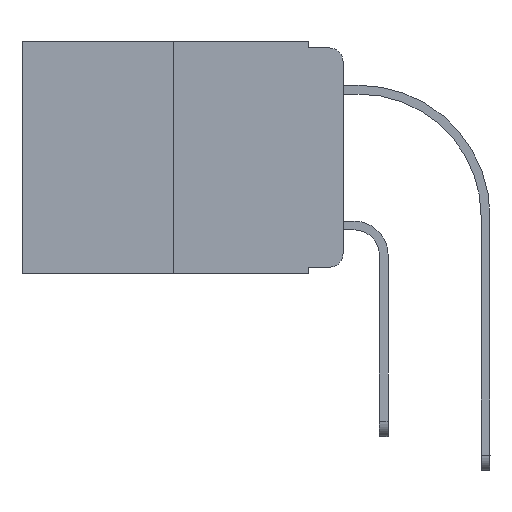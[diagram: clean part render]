
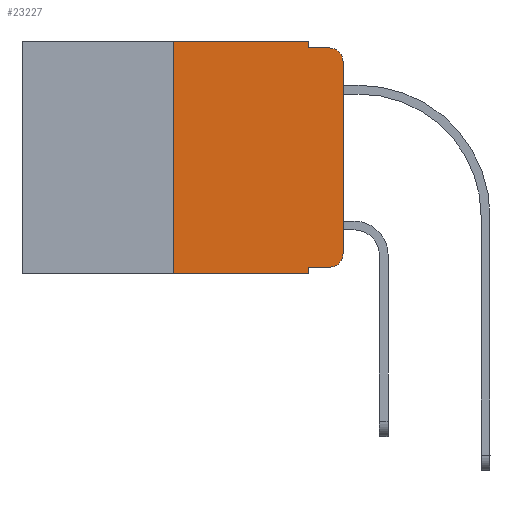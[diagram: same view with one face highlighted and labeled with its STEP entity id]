
A CAD part, left-side view. The second image highlights one B-rep face of the part: STEP entity #23227.
In plain terms, the highlighted planar face has unit normal (-1, 0, 0).
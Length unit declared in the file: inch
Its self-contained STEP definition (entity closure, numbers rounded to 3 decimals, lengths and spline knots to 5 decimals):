
#122 = EDGE_CURVE ( 'NONE', #24338, #26488, #23651, .T. ) ;
#139 = CARTESIAN_POINT ( 'NONE',  ( 0., 0.051, -0.01 ) ) ;
#524 = CARTESIAN_POINT ( 'NONE',  ( 0., 0.051, -0.01 ) ) ;
#1080 = CARTESIAN_POINT ( 'NONE',  ( 0., 0.473, 0. ) ) ;
#1432 = DIRECTION ( 'NONE',  ( 0., 0., -1. ) ) ;
#1487 = DIRECTION ( 'NONE',  ( 0., -1., 0. ) ) ;
#1565 = VECTOR ( 'NONE', #1432, 39.37008 ) ;
#1876 = DIRECTION ( 'NONE',  ( 0., 0., 1. ) ) ;
#2195 = EDGE_CURVE ( 'NONE', #5701, #9958, #22381, .T. ) ;
#2500 = VERTEX_POINT ( 'NONE', #13990 ) ;
#2612 = DIRECTION ( 'NONE',  ( 0., -1., 0. ) ) ;
#3319 = CARTESIAN_POINT ( 'NONE',  ( 0., 0.25, 0. ) ) ;
#3854 = CARTESIAN_POINT ( 'NONE',  ( 0., 0., -0.313 ) ) ;
#4149 = VERTEX_POINT ( 'NONE', #12346 ) ;
#4293 = EDGE_CURVE ( 'NONE', #4149, #24338, #19023, .T. ) ;
#4518 = CIRCLE ( 'NONE', #11486, 0.02 ) ;
#4708 = LINE ( 'NONE', #25182, #15125 ) ;
#5687 = EDGE_CURVE ( 'NONE', #6846, #24163, #4518, .T. ) ;
#5701 = VERTEX_POINT ( 'NONE', #9592 ) ;
#6397 = DIRECTION ( 'NONE',  ( 0., -1., 0. ) ) ;
#6399 = ORIENTED_EDGE ( 'NONE', *, *, #12714, .F. ) ;
#6846 = VERTEX_POINT ( 'NONE', #12774 ) ;
#7300 = DIRECTION ( 'NONE',  ( 0., 0., 1. ) ) ;
#7724 = ORIENTED_EDGE ( 'NONE', *, *, #22183, .T. ) ;
#7801 = VERTEX_POINT ( 'NONE', #10499 ) ;
#7982 = EDGE_LOOP ( 'NONE', ( #13857, #7724, #8784, #21289, #6399, #9930, #16809, #25995, #10051, #22734 ) ) ;
#8472 = VECTOR ( 'NONE', #7300, 39.37008 ) ;
#8784 = ORIENTED_EDGE ( 'NONE', *, *, #122, .F. ) ;
#9409 = DIRECTION ( 'NONE',  ( 1., 0., 0. ) ) ;
#9592 = CARTESIAN_POINT ( 'NONE',  ( 0., 0.25, -0.343 ) ) ;
#9930 = ORIENTED_EDGE ( 'NONE', *, *, #14198, .F. ) ;
#9958 = VERTEX_POINT ( 'NONE', #18833 ) ;
#10037 = DIRECTION ( 'NONE',  ( -1., 0., 0. ) ) ;
#10051 = ORIENTED_EDGE ( 'NONE', *, *, #18246, .T. ) ;
#10071 = CARTESIAN_POINT ( 'NONE',  ( 0., 0.473, -0.343 ) ) ;
#10430 = DIRECTION ( 'NONE',  ( 0., 0., -1. ) ) ;
#10499 = CARTESIAN_POINT ( 'NONE',  ( 0., 0.25, 0. ) ) ;
#10793 = CARTESIAN_POINT ( 'NONE',  ( 0., 0.051, -0.333 ) ) ;
#11015 = EDGE_CURVE ( 'NONE', #13066, #9958, #26423, .T. ) ;
#11486 = AXIS2_PLACEMENT_3D ( 'NONE', #25319, #14923, #14803 ) ;
#12346 = CARTESIAN_POINT ( 'NONE',  ( 0., 0.051, 0. ) ) ;
#12363 = CARTESIAN_POINT ( 'NONE',  ( 0., 0.02, -0.03 ) ) ;
#12500 = VECTOR ( 'NONE', #6397, 39.37008 ) ;
#12528 = LINE ( 'NONE', #18531, #12500 ) ;
#12714 = EDGE_CURVE ( 'NONE', #7801, #4149, #4708, .T. ) ;
#12774 = CARTESIAN_POINT ( 'NONE',  ( 0., 0.02, -0.333 ) ) ;
#13066 = VERTEX_POINT ( 'NONE', #10793 ) ;
#13857 = ORIENTED_EDGE ( 'NONE', *, *, #18279, .T. ) ;
#13990 = CARTESIAN_POINT ( 'NONE',  ( 0., 0., -0.03 ) ) ;
#14147 = DIRECTION ( 'NONE',  ( 0., 0., -1. ) ) ;
#14198 = EDGE_CURVE ( 'NONE', #5701, #7801, #22038, .T. ) ;
#14682 = VECTOR ( 'NONE', #1876, 39.37008 ) ;
#14803 = DIRECTION ( 'NONE',  ( 0., 0., -1. ) ) ;
#14917 = CARTESIAN_POINT ( 'NONE',  ( 0., 0.051, 0. ) ) ;
#14923 = DIRECTION ( 'NONE',  ( -1., 0., 0. ) ) ;
#15125 = VECTOR ( 'NONE', #25988, 39.37008 ) ;
#15651 = CIRCLE ( 'NONE', #21790, 0.02 ) ;
#15767 = VECTOR ( 'NONE', #1487, 39.37008 ) ;
#16355 = CARTESIAN_POINT ( 'NONE',  ( 0., 0., 0. ) ) ;
#16360 = CARTESIAN_POINT ( 'NONE',  ( 0., 0.02, -0.01 ) ) ;
#16708 = VECTOR ( 'NONE', #10430, 39.37008 ) ;
#16809 = ORIENTED_EDGE ( 'NONE', *, *, #2195, .T. ) ;
#18246 = EDGE_CURVE ( 'NONE', #13066, #6846, #12528, .T. ) ;
#18279 = EDGE_CURVE ( 'NONE', #24163, #2500, #22648, .T. ) ;
#18531 = CARTESIAN_POINT ( 'NONE',  ( 0., 0.051, -0.333 ) ) ;
#18833 = CARTESIAN_POINT ( 'NONE',  ( 0., 0.051, -0.343 ) ) ;
#19023 = LINE ( 'NONE', #14917, #16708 ) ;
#19651 = FACE_OUTER_BOUND ( 'NONE', #7982, .T. ) ;
#21289 = ORIENTED_EDGE ( 'NONE', *, *, #4293, .F. ) ;
#21790 = AXIS2_PLACEMENT_3D ( 'NONE', #12363, #10037, #14147 ) ;
#22038 = LINE ( 'NONE', #3319, #8472 ) ;
#22124 = PLANE ( 'NONE',  #24870 ) ;
#22183 = EDGE_CURVE ( 'NONE', #2500, #26488, #15651, .T. ) ;
#22381 = LINE ( 'NONE', #10071, #15767 ) ;
#22648 = LINE ( 'NONE', #16355, #14682 ) ;
#22734 = ORIENTED_EDGE ( 'NONE', *, *, #5687, .T. ) ;
#23227 = ADVANCED_FACE ( 'NONE', ( #19651 ), #22124, .F. ) ;
#23651 = LINE ( 'NONE', #139, #25824 ) ;
#24163 = VERTEX_POINT ( 'NONE', #3854 ) ;
#24338 = VERTEX_POINT ( 'NONE', #524 ) ;
#24870 = AXIS2_PLACEMENT_3D ( 'NONE', #1080, #9409, #26076 ) ;
#25182 = CARTESIAN_POINT ( 'NONE',  ( 0., 0.473, 0. ) ) ;
#25319 = CARTESIAN_POINT ( 'NONE',  ( 0., 0.02, -0.313 ) ) ;
#25824 = VECTOR ( 'NONE', #2612, 39.37008 ) ;
#25988 = DIRECTION ( 'NONE',  ( 0., -1., 0. ) ) ;
#25995 = ORIENTED_EDGE ( 'NONE', *, *, #11015, .F. ) ;
#26076 = DIRECTION ( 'NONE',  ( 0., 0., -1. ) ) ;
#26274 = CARTESIAN_POINT ( 'NONE',  ( 0., 0.051, 0. ) ) ;
#26423 = LINE ( 'NONE', #26274, #1565 ) ;
#26488 = VERTEX_POINT ( 'NONE', #16360 ) ;
